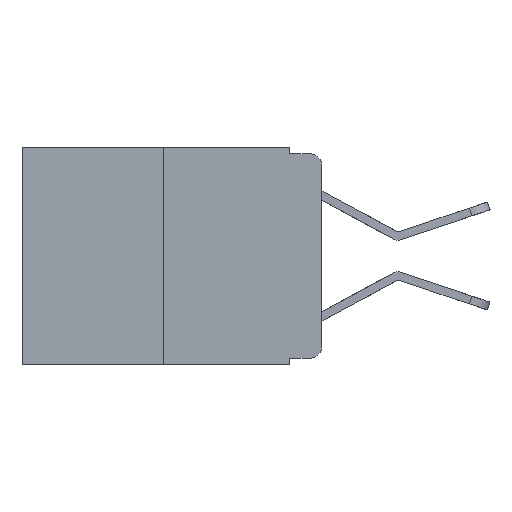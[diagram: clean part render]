
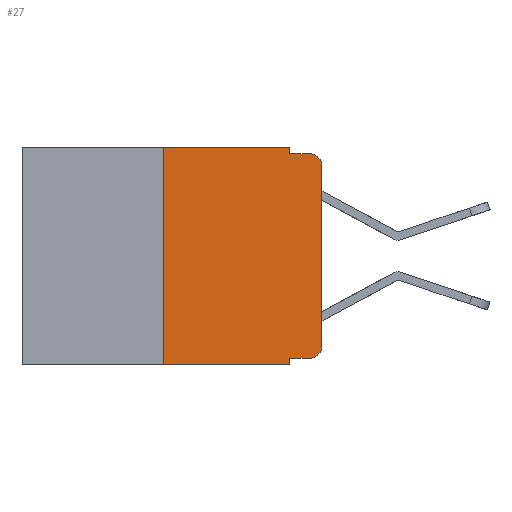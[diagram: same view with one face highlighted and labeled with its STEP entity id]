
A CAD part, left-side view. The second image highlights one B-rep face of the part: STEP entity #27.
In plain terms, the highlighted planar face has unit normal (-1, 0, 0).
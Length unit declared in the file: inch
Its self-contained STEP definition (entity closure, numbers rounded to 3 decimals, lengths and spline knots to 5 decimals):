
#17 = VECTOR ( 'NONE', #9052, 39.37008 ) ;
#27 = ADVANCED_FACE ( 'NONE', ( #9096 ), #9499, .F. ) ;
#29 = CARTESIAN_POINT ( 'NONE',  ( 0., 0.25, 0. ) ) ;
#361 = VERTEX_POINT ( 'NONE', #4161 ) ;
#569 = VERTEX_POINT ( 'NONE', #7538 ) ;
#599 = EDGE_CURVE ( 'NONE', #3653, #4874, #5464, .T. ) ;
#921 = DIRECTION ( 'NONE',  ( 0., 0., -1. ) ) ;
#1451 = LINE ( 'NONE', #3617, #11125 ) ;
#1627 = DIRECTION ( 'NONE',  ( 0., 0., 1. ) ) ;
#1979 = CARTESIAN_POINT ( 'NONE',  ( 0., 0.02, -0.313 ) ) ;
#2067 = DIRECTION ( 'NONE',  ( 1., 0., 0. ) ) ;
#2425 = LINE ( 'NONE', #7111, #9412 ) ;
#2460 = DIRECTION ( 'NONE',  ( 0., -1., 0. ) ) ;
#2755 = CARTESIAN_POINT ( 'NONE',  ( 0., 0.051, -0.01 ) ) ;
#2822 = DIRECTION ( 'NONE',  ( 0., 0., 1. ) ) ;
#2855 = LINE ( 'NONE', #6328, #17 ) ;
#2978 = DIRECTION ( 'NONE',  ( 0., 0., -1. ) ) ;
#3025 = VERTEX_POINT ( 'NONE', #10396 ) ;
#3187 = ORIENTED_EDGE ( 'NONE', *, *, #10424, .F. ) ;
#3334 = CARTESIAN_POINT ( 'NONE',  ( 0., 0.02, -0.03 ) ) ;
#3418 = VERTEX_POINT ( 'NONE', #4339 ) ;
#3595 = DIRECTION ( 'NONE',  ( 0., -1., 0. ) ) ;
#3617 = CARTESIAN_POINT ( 'NONE',  ( 0., 0.25, 0. ) ) ;
#3653 = VERTEX_POINT ( 'NONE', #7436 ) ;
#3748 = EDGE_CURVE ( 'NONE', #3025, #361, #5282, .T. ) ;
#3837 = CARTESIAN_POINT ( 'NONE',  ( 0., 0., -0.03 ) ) ;
#3939 = ORIENTED_EDGE ( 'NONE', *, *, #3748, .T. ) ;
#4161 = CARTESIAN_POINT ( 'NONE',  ( 0., 0.051, -0.343 ) ) ;
#4183 = ORIENTED_EDGE ( 'NONE', *, *, #5248, .F. ) ;
#4204 = CARTESIAN_POINT ( 'NONE',  ( 0., 0.051, -0.333 ) ) ;
#4314 = DIRECTION ( 'NONE',  ( 0., 0., -1. ) ) ;
#4333 = VERTEX_POINT ( 'NONE', #4204 ) ;
#4339 = CARTESIAN_POINT ( 'NONE',  ( 0., 0.02, -0.01 ) ) ;
#4772 = EDGE_LOOP ( 'NONE', ( #8238, #12250, #5196, #3187, #4183, #10198, #3939, #10462, #5213, #11557 ) ) ;
#4874 = VERTEX_POINT ( 'NONE', #3837 ) ;
#5196 = ORIENTED_EDGE ( 'NONE', *, *, #11001, .F. ) ;
#5213 = ORIENTED_EDGE ( 'NONE', *, *, #8712, .T. ) ;
#5248 = EDGE_CURVE ( 'NONE', #11466, #569, #11722, .T. ) ;
#5282 = LINE ( 'NONE', #6515, #9859 ) ;
#5464 = LINE ( 'NONE', #9629, #12041 ) ;
#5501 = VERTEX_POINT ( 'NONE', #2755 ) ;
#5687 = CARTESIAN_POINT ( 'NONE',  ( 0., 0.02, -0.333 ) ) ;
#5755 = DIRECTION ( 'NONE',  ( 0., 0., -1. ) ) ;
#5915 = CARTESIAN_POINT ( 'NONE',  ( 0., 0.051, 0. ) ) ;
#6257 = CIRCLE ( 'NONE', #6756, 0.02 ) ;
#6328 = CARTESIAN_POINT ( 'NONE',  ( 0., 0.051, 0. ) ) ;
#6410 = CARTESIAN_POINT ( 'NONE',  ( 0., 0.473, 0. ) ) ;
#6459 = VECTOR ( 'NONE', #921, 39.37008 ) ;
#6515 = CARTESIAN_POINT ( 'NONE',  ( 0., 0.473, -0.343 ) ) ;
#6586 = CARTESIAN_POINT ( 'NONE',  ( 0., 0.051, -0.01 ) ) ;
#6756 = AXIS2_PLACEMENT_3D ( 'NONE', #3334, #9879, #4314 ) ;
#6895 = AXIS2_PLACEMENT_3D ( 'NONE', #1979, #8715, #2978 ) ;
#7111 = CARTESIAN_POINT ( 'NONE',  ( 0., 0.051, -0.333 ) ) ;
#7436 = CARTESIAN_POINT ( 'NONE',  ( 0., 0., -0.313 ) ) ;
#7538 = CARTESIAN_POINT ( 'NONE',  ( 0., 0.051, 0. ) ) ;
#7947 = CIRCLE ( 'NONE', #6895, 0.02 ) ;
#8147 = EDGE_CURVE ( 'NONE', #9098, #3653, #7947, .T. ) ;
#8238 = ORIENTED_EDGE ( 'NONE', *, *, #599, .T. ) ;
#8712 = EDGE_CURVE ( 'NONE', #4333, #9098, #2425, .T. ) ;
#8715 = DIRECTION ( 'NONE',  ( -1., 0., 0. ) ) ;
#8863 = LINE ( 'NONE', #5915, #6459 ) ;
#8959 = VECTOR ( 'NONE', #3595, 39.37008 ) ;
#9052 = DIRECTION ( 'NONE',  ( 0., 0., -1. ) ) ;
#9096 = FACE_OUTER_BOUND ( 'NONE', #4772, .T. ) ;
#9098 = VERTEX_POINT ( 'NONE', #5687 ) ;
#9275 = EDGE_CURVE ( 'NONE', #4333, #361, #8863, .T. ) ;
#9412 = VECTOR ( 'NONE', #11482, 39.37008 ) ;
#9499 = PLANE ( 'NONE',  #12203 ) ;
#9629 = CARTESIAN_POINT ( 'NONE',  ( 0., 0., 0. ) ) ;
#9692 = VECTOR ( 'NONE', #2460, 39.37008 ) ;
#9751 = CARTESIAN_POINT ( 'NONE',  ( 0., 0.473, 0. ) ) ;
#9842 = EDGE_CURVE ( 'NONE', #3025, #11466, #1451, .T. ) ;
#9859 = VECTOR ( 'NONE', #10706, 39.37008 ) ;
#9879 = DIRECTION ( 'NONE',  ( -1., 0., 0. ) ) ;
#10198 = ORIENTED_EDGE ( 'NONE', *, *, #9842, .F. ) ;
#10396 = CARTESIAN_POINT ( 'NONE',  ( 0., 0.25, -0.343 ) ) ;
#10424 = EDGE_CURVE ( 'NONE', #569, #5501, #2855, .T. ) ;
#10462 = ORIENTED_EDGE ( 'NONE', *, *, #9275, .F. ) ;
#10706 = DIRECTION ( 'NONE',  ( 0., -1., 0. ) ) ;
#11001 = EDGE_CURVE ( 'NONE', #5501, #3418, #11237, .T. ) ;
#11125 = VECTOR ( 'NONE', #1627, 39.37008 ) ;
#11237 = LINE ( 'NONE', #6586, #8959 ) ;
#11466 = VERTEX_POINT ( 'NONE', #29 ) ;
#11482 = DIRECTION ( 'NONE',  ( 0., -1., 0. ) ) ;
#11557 = ORIENTED_EDGE ( 'NONE', *, *, #8147, .T. ) ;
#11580 = EDGE_CURVE ( 'NONE', #4874, #3418, #6257, .T. ) ;
#11722 = LINE ( 'NONE', #6410, #9692 ) ;
#12041 = VECTOR ( 'NONE', #2822, 39.37008 ) ;
#12203 = AXIS2_PLACEMENT_3D ( 'NONE', #9751, #2067, #5755 ) ;
#12250 = ORIENTED_EDGE ( 'NONE', *, *, #11580, .T. ) ;
